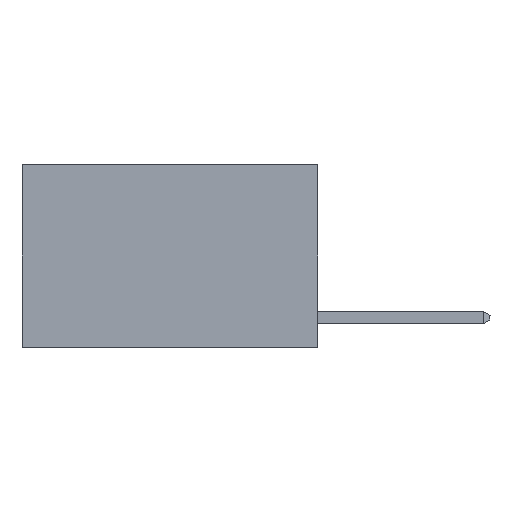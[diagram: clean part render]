
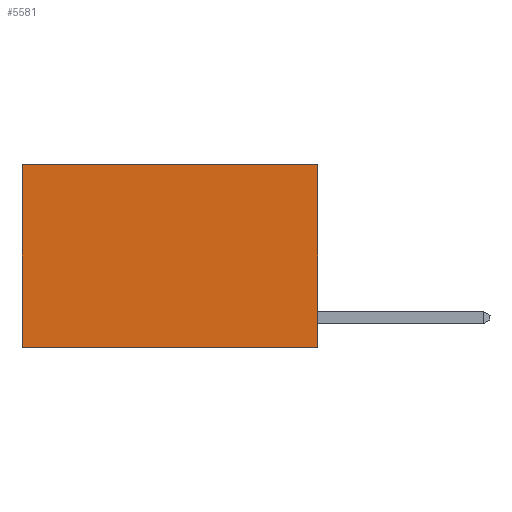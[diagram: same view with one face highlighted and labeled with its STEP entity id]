
A CAD part, left-side view. The second image highlights one B-rep face of the part: STEP entity #5581.
In plain terms, the highlighted planar face has unit normal (-1, 0, 0).
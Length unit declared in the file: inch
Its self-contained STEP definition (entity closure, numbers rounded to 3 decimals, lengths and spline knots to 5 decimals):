
#3340 = DIRECTION ( 'NONE',  ( 1., 0., 0. ) ) ;
#3346 = AXIS2_PLACEMENT_3D ( 'NONE', #10606, #3340, #4569 ) ;
#3677 = CARTESIAN_POINT ( 'NONE',  ( 0.2625, 0., 0. ) ) ;
#3827 = ORIENTED_EDGE ( 'NONE', *, *, #12426, .T. ) ;
#4202 = VECTOR ( 'NONE', #13069, 39.37008 ) ;
#4569 = DIRECTION ( 'NONE',  ( 0., 0., -1. ) ) ;
#4607 = CARTESIAN_POINT ( 'NONE',  ( 0.2625, 0.6, 0. ) ) ;
#4958 = CARTESIAN_POINT ( 'NONE',  ( 0.2625, 0., -0.37 ) ) ;
#4970 = VERTEX_POINT ( 'NONE', #9279 ) ;
#5458 = EDGE_CURVE ( 'NONE', #8347, #13667, #11733, .T. ) ;
#5581 = ADVANCED_FACE ( 'NONE', ( #9841 ), #11798, .F. ) ;
#5615 = EDGE_CURVE ( 'NONE', #12199, #4970, #13053, .T. ) ;
#6445 = LINE ( 'NONE', #3677, #13072 ) ;
#6620 = VECTOR ( 'NONE', #14450, 39.37008 ) ;
#6685 = DIRECTION ( 'NONE',  ( 0., 1., 0. ) ) ;
#7023 = EDGE_CURVE ( 'NONE', #8347, #12199, #6445, .T. ) ;
#7569 = CARTESIAN_POINT ( 'NONE',  ( 0.2625, 0., -0.37 ) ) ;
#7927 = ORIENTED_EDGE ( 'NONE', *, *, #5615, .F. ) ;
#8347 = VERTEX_POINT ( 'NONE', #14623 ) ;
#8529 = VECTOR ( 'NONE', #6685, 39.37008 ) ;
#8999 = EDGE_LOOP ( 'NONE', ( #3827, #7927, #14867, #10643 ) ) ;
#9279 = CARTESIAN_POINT ( 'NONE',  ( 0.2625, 0.6, -0.37 ) ) ;
#9841 = FACE_OUTER_BOUND ( 'NONE', #8999, .T. ) ;
#10606 = CARTESIAN_POINT ( 'NONE',  ( 0.2625, 0., 0. ) ) ;
#10643 = ORIENTED_EDGE ( 'NONE', *, *, #5458, .T. ) ;
#10712 = CARTESIAN_POINT ( 'NONE',  ( 0.2625, 0.6, 0. ) ) ;
#11733 = LINE ( 'NONE', #12558, #8529 ) ;
#11798 = PLANE ( 'NONE',  #3346 ) ;
#11966 = DIRECTION ( 'NONE',  ( 0., 0., -1. ) ) ;
#12199 = VERTEX_POINT ( 'NONE', #7569 ) ;
#12426 = EDGE_CURVE ( 'NONE', #13667, #4970, #13664, .T. ) ;
#12558 = CARTESIAN_POINT ( 'NONE',  ( 0.2625, 0., 0. ) ) ;
#13053 = LINE ( 'NONE', #4958, #6620 ) ;
#13069 = DIRECTION ( 'NONE',  ( 0., 0., -1. ) ) ;
#13072 = VECTOR ( 'NONE', #11966, 39.37008 ) ;
#13664 = LINE ( 'NONE', #4607, #4202 ) ;
#13667 = VERTEX_POINT ( 'NONE', #10712 ) ;
#14450 = DIRECTION ( 'NONE',  ( 0., 1., 0. ) ) ;
#14623 = CARTESIAN_POINT ( 'NONE',  ( 0.2625, 0., 0. ) ) ;
#14867 = ORIENTED_EDGE ( 'NONE', *, *, #7023, .F. ) ;
